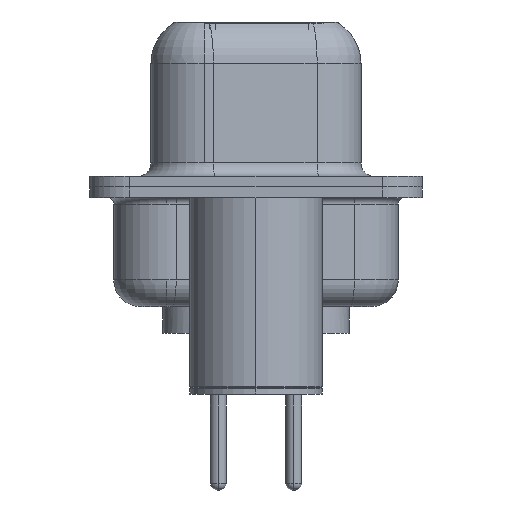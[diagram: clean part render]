
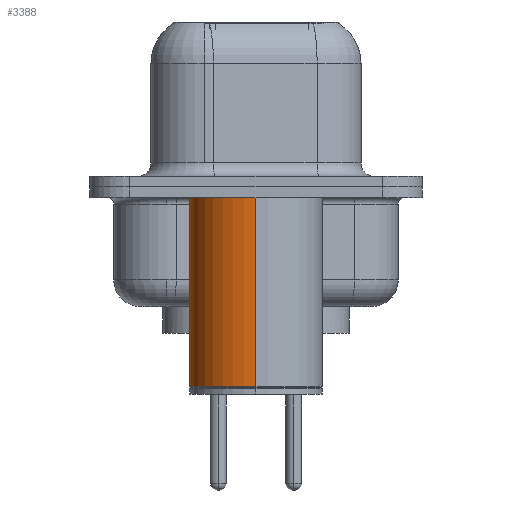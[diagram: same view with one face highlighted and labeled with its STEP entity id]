
A CAD part, left-side view. The second image highlights one B-rep face of the part: STEP entity #3388.
In plain terms, the highlighted cylindrical face has radius 2.5 mm (diameter 5 mm), a partial arc.
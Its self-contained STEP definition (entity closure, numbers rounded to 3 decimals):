
#781 = VECTOR ( 'NONE', #23519, 1000. ) ;
#1407 = DIRECTION ( 'NONE',  ( 0., 0., 1. ) ) ;
#1699 = ORIENTED_EDGE ( 'NONE', *, *, #4681, .T. ) ;
#1761 = DIRECTION ( 'NONE',  ( 0., 0., 1. ) ) ;
#2081 = CARTESIAN_POINT ( 'NONE',  ( 2.5, 0., -0.4 ) ) ;
#3185 = ORIENTED_EDGE ( 'NONE', *, *, #5011, .F. ) ;
#3388 = ADVANCED_FACE ( 'NONE', ( #20369 ), #24772, .T. ) ;
#4186 = VERTEX_POINT ( 'NONE', #25088 ) ;
#4681 = EDGE_CURVE ( 'NONE', #5228, #4186, #10427, .T. ) ;
#4954 = DIRECTION ( 'NONE',  ( 1., 0., 0. ) ) ;
#5011 = EDGE_CURVE ( 'NONE', #5228, #27040, #6452, .T. ) ;
#5228 = VERTEX_POINT ( 'NONE', #23929 ) ;
#6452 = LINE ( 'NONE', #14876, #781 ) ;
#7862 = CARTESIAN_POINT ( 'NONE',  ( -2.5, 0., 0.581 ) ) ;
#8092 = AXIS2_PLACEMENT_3D ( 'NONE', #14313, #1761, #10158 ) ;
#8580 = CARTESIAN_POINT ( 'NONE',  ( -2.5, 0., -0.4 ) ) ;
#9472 = AXIS2_PLACEMENT_3D ( 'NONE', #10577, #10867, #14851 ) ;
#9495 = CARTESIAN_POINT ( 'NONE',  ( 0., 0., -7.525 ) ) ;
#10158 = DIRECTION ( 'NONE',  ( 1., 0., 0. ) ) ;
#10427 = CIRCLE ( 'NONE', #21405, 2.5 ) ;
#10577 = CARTESIAN_POINT ( 'NONE',  ( 0., 0., -0.4 ) ) ;
#10867 = DIRECTION ( 'NONE',  ( 0., 0., 1. ) ) ;
#14313 = CARTESIAN_POINT ( 'NONE',  ( 0., 0., 0.581 ) ) ;
#14398 = ORIENTED_EDGE ( 'NONE', *, *, #14742, .T. ) ;
#14742 = EDGE_CURVE ( 'NONE', #4186, #14986, #15894, .T. ) ;
#14851 = DIRECTION ( 'NONE',  ( 1., 0., 0. ) ) ;
#14876 = CARTESIAN_POINT ( 'NONE',  ( 2.5, 0., 0.581 ) ) ;
#14986 = VERTEX_POINT ( 'NONE', #8580 ) ;
#15894 = LINE ( 'NONE', #7862, #24712 ) ;
#16419 = EDGE_LOOP ( 'NONE', ( #1699, #14398, #18324, #3185 ) ) ;
#18324 = ORIENTED_EDGE ( 'NONE', *, *, #19060, .F. ) ;
#19060 = EDGE_CURVE ( 'NONE', #27040, #14986, #21363, .T. ) ;
#20369 = FACE_OUTER_BOUND ( 'NONE', #16419, .T. ) ;
#21363 = CIRCLE ( 'NONE', #9472, 2.5 ) ;
#21405 = AXIS2_PLACEMENT_3D ( 'NONE', #9495, #24097, #4954 ) ;
#23519 = DIRECTION ( 'NONE',  ( 0., 0., 1. ) ) ;
#23929 = CARTESIAN_POINT ( 'NONE',  ( 2.5, 0., -7.525 ) ) ;
#24097 = DIRECTION ( 'NONE',  ( 0., 0., 1. ) ) ;
#24712 = VECTOR ( 'NONE', #1407, 1000. ) ;
#24772 = CYLINDRICAL_SURFACE ( 'NONE', #8092, 2.5 ) ;
#25088 = CARTESIAN_POINT ( 'NONE',  ( -2.5, 0., -7.525 ) ) ;
#27040 = VERTEX_POINT ( 'NONE', #2081 ) ;
